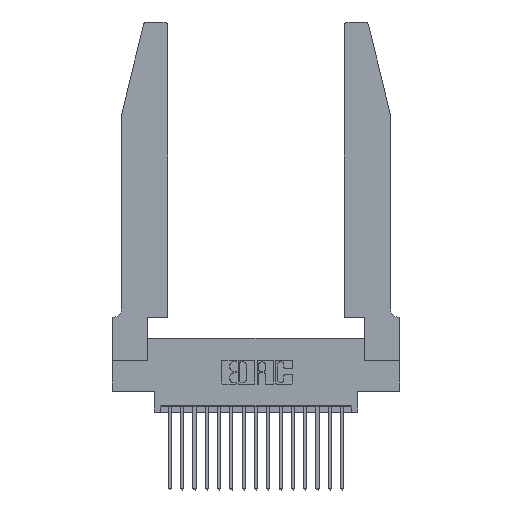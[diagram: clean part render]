
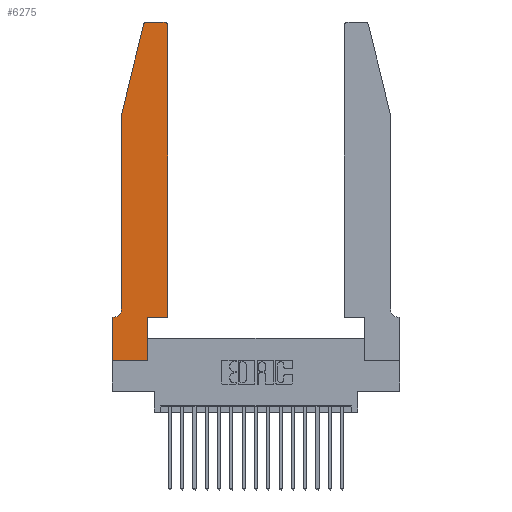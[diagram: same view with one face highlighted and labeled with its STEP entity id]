
A CAD part, top view. The second image highlights one B-rep face of the part: STEP entity #6275.
In plain terms, the highlighted planar face has unit normal (0, 0, 1).
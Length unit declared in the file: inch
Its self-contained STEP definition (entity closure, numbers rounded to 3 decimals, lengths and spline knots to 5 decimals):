
#132 = LINE ( 'NONE', #19241, #16407 ) ;
#251 = DIRECTION ( 'NONE',  ( -0.239, -0.971, 0. ) ) ;
#421 = ORIENTED_EDGE ( 'NONE', *, *, #3381, .T. ) ;
#512 = VECTOR ( 'NONE', #2416, 39.37008 ) ;
#868 = EDGE_CURVE ( 'NONE', #13616, #20068, #10272, .T. ) ;
#911 = ORIENTED_EDGE ( 'NONE', *, *, #13147, .T. ) ;
#1141 = EDGE_CURVE ( 'NONE', #5732, #8431, #18266, .T. ) ;
#1251 = CARTESIAN_POINT ( 'NONE',  ( 0.4205, 2.75, 0.37 ) ) ;
#1367 = VERTEX_POINT ( 'NONE', #13797 ) ;
#1369 = CARTESIAN_POINT ( 'NONE',  ( 0.4505, 0.35, 0.37 ) ) ;
#1503 = EDGE_CURVE ( 'NONE', #18216, #5732, #12931, .T. ) ;
#2416 = DIRECTION ( 'NONE',  ( 0., 1., 0. ) ) ;
#2422 = ORIENTED_EDGE ( 'NONE', *, *, #7272, .T. ) ;
#2637 = VERTEX_POINT ( 'NONE', #19944 ) ;
#2815 = CARTESIAN_POINT ( 'NONE',  ( 0.284, 2.75, 0.37 ) ) ;
#2861 = CARTESIAN_POINT ( 'NONE',  ( 0., 0.35, 0.37 ) ) ;
#2980 = VERTEX_POINT ( 'NONE', #4996 ) ;
#3059 = CARTESIAN_POINT ( 'NONE',  ( 0.0055, 0.42, 0.37 ) ) ;
#3167 = CARTESIAN_POINT ( 'NONE',  ( 0., 0.35, 0.37 ) ) ;
#3179 = ORIENTED_EDGE ( 'NONE', *, *, #16880, .T. ) ;
#3381 = EDGE_CURVE ( 'NONE', #19368, #2980, #3508, .T. ) ;
#3508 = LINE ( 'NONE', #18440, #19646 ) ;
#3659 = DIRECTION ( 'NONE',  ( 0., -1., 0. ) ) ;
#4074 = EDGE_CURVE ( 'NONE', #2980, #18216, #18404, .T. ) ;
#4141 = CARTESIAN_POINT ( 'NONE',  ( 0., 0., 0.37 ) ) ;
#4421 = ORIENTED_EDGE ( 'NONE', *, *, #868, .T. ) ;
#4464 = EDGE_CURVE ( 'NONE', #18987, #2637, #7931, .T. ) ;
#4649 = DIRECTION ( 'NONE',  ( -1., 0., 0. ) ) ;
#4820 = DIRECTION ( 'NONE',  ( 1., 0., 0. ) ) ;
#4996 = CARTESIAN_POINT ( 'NONE',  ( 0.4505, 2.72, 0.37 ) ) ;
#5023 = DIRECTION ( 'NONE',  ( 0., 0., 1. ) ) ;
#5327 = AXIS2_PLACEMENT_3D ( 'NONE', #14456, #5023, #15990 ) ;
#5559 = CARTESIAN_POINT ( 'NONE',  ( 0.0755, 0.35, 0.37 ) ) ;
#5666 = CARTESIAN_POINT ( 'NONE',  ( 0.2865, 0.35, 0.37 ) ) ;
#5732 = VERTEX_POINT ( 'NONE', #2815 ) ;
#6086 = PLANE ( 'NONE',  #13521 ) ;
#6092 = VECTOR ( 'NONE', #13229, 39.37008 ) ;
#6275 = ADVANCED_FACE ( 'NONE', ( #7425 ), #6086, .T. ) ;
#6898 = VECTOR ( 'NONE', #17969, 39.37008 ) ;
#7006 = EDGE_CURVE ( 'NONE', #8628, #19368, #7628, .T. ) ;
#7205 = CARTESIAN_POINT ( 'NONE',  ( 0.0755, 2., 0.37 ) ) ;
#7272 = EDGE_CURVE ( 'NONE', #2637, #13616, #19769, .T. ) ;
#7425 = FACE_OUTER_BOUND ( 'NONE', #13802, .T. ) ;
#7575 = DIRECTION ( 'NONE',  ( 0., 1., 0. ) ) ;
#7628 = LINE ( 'NONE', #1369, #20007 ) ;
#7666 = DIRECTION ( 'NONE',  ( 0., 0., 1. ) ) ;
#7931 = CIRCLE ( 'NONE', #10238, 0.07 ) ;
#8431 = VERTEX_POINT ( 'NONE', #14666 ) ;
#8628 = VERTEX_POINT ( 'NONE', #5666 ) ;
#8636 = CARTESIAN_POINT ( 'NONE',  ( 0.284, 2.72, 0.37 ) ) ;
#8788 = VECTOR ( 'NONE', #18674, 39.37008 ) ;
#8901 = ORIENTED_EDGE ( 'NONE', *, *, #4074, .T. ) ;
#9200 = DIRECTION ( 'NONE',  ( 0., 0., 1. ) ) ;
#10238 = AXIS2_PLACEMENT_3D ( 'NONE', #3059, #14094, #4649 ) ;
#10272 = LINE ( 'NONE', #15895, #6092 ) ;
#10351 = ORIENTED_EDGE ( 'NONE', *, *, #4464, .T. ) ;
#10864 = VECTOR ( 'NONE', #11062, 39.37008 ) ;
#10868 = DIRECTION ( 'NONE',  ( 1., 0., 0. ) ) ;
#11062 = DIRECTION ( 'NONE',  ( 1., 0., 0. ) ) ;
#11335 = LINE ( 'NONE', #12915, #19082 ) ;
#11890 = CARTESIAN_POINT ( 'NONE',  ( 0.2865, 0.35, 0.37 ) ) ;
#12915 = CARTESIAN_POINT ( 'NONE',  ( 0.0755, 2., 0.37 ) ) ;
#12931 = LINE ( 'NONE', #13414, #8788 ) ;
#13147 = EDGE_CURVE ( 'NONE', #8431, #14885, #11335, .T. ) ;
#13229 = DIRECTION ( 'NONE',  ( 0., -1., 0. ) ) ;
#13414 = CARTESIAN_POINT ( 'NONE',  ( 0.2605, 2.75, 0.37 ) ) ;
#13521 = AXIS2_PLACEMENT_3D ( 'NONE', #2861, #7666, #18542 ) ;
#13616 = VERTEX_POINT ( 'NONE', #3167 ) ;
#13797 = CARTESIAN_POINT ( 'NONE',  ( 0.2865, 0., 0.37 ) ) ;
#13802 = EDGE_LOOP ( 'NONE', ( #14254, #19310, #911, #14015, #10351, #2422, #4421, #17393, #3179, #16211, #421, #8901 ) ) ;
#13988 = EDGE_CURVE ( 'NONE', #14885, #18987, #132, .T. ) ;
#14015 = ORIENTED_EDGE ( 'NONE', *, *, #13988, .T. ) ;
#14094 = DIRECTION ( 'NONE',  ( 0., 0., -1. ) ) ;
#14254 = ORIENTED_EDGE ( 'NONE', *, *, #1503, .T. ) ;
#14456 = CARTESIAN_POINT ( 'NONE',  ( 0.4205, 2.72, 0.37 ) ) ;
#14666 = CARTESIAN_POINT ( 'NONE',  ( 0.25487, 2.72718, 0.37 ) ) ;
#14885 = VERTEX_POINT ( 'NONE', #7205 ) ;
#15014 = LINE ( 'NONE', #17228, #10864 ) ;
#15167 = AXIS2_PLACEMENT_3D ( 'NONE', #8636, #9200, #4820 ) ;
#15895 = CARTESIAN_POINT ( 'NONE',  ( 0., 0., 0.37 ) ) ;
#15990 = DIRECTION ( 'NONE',  ( 1., 0., 0. ) ) ;
#16211 = ORIENTED_EDGE ( 'NONE', *, *, #7006, .T. ) ;
#16299 = LINE ( 'NONE', #11890, #512 ) ;
#16407 = VECTOR ( 'NONE', #3659, 39.37008 ) ;
#16478 = CARTESIAN_POINT ( 'NONE',  ( 0.4505, 0.35, 0.37 ) ) ;
#16880 = EDGE_CURVE ( 'NONE', #1367, #8628, #16299, .T. ) ;
#17165 = CARTESIAN_POINT ( 'NONE',  ( 0.0755, 0.42, 0.37 ) ) ;
#17228 = CARTESIAN_POINT ( 'NONE',  ( 0., 0., 0.37 ) ) ;
#17393 = ORIENTED_EDGE ( 'NONE', *, *, #19805, .T. ) ;
#17969 = DIRECTION ( 'NONE',  ( -1., 0., 0. ) ) ;
#18216 = VERTEX_POINT ( 'NONE', #1251 ) ;
#18266 = CIRCLE ( 'NONE', #15167, 0.03 ) ;
#18404 = CIRCLE ( 'NONE', #5327, 0.03 ) ;
#18440 = CARTESIAN_POINT ( 'NONE',  ( 0.4505, 0.35, 0.37 ) ) ;
#18542 = DIRECTION ( 'NONE',  ( 1., 0., 0. ) ) ;
#18674 = DIRECTION ( 'NONE',  ( -1., 0., 0. ) ) ;
#18987 = VERTEX_POINT ( 'NONE', #17165 ) ;
#19082 = VECTOR ( 'NONE', #251, 39.37008 ) ;
#19241 = CARTESIAN_POINT ( 'NONE',  ( 0.0755, 2., 0.37 ) ) ;
#19310 = ORIENTED_EDGE ( 'NONE', *, *, #1141, .T. ) ;
#19368 = VERTEX_POINT ( 'NONE', #16478 ) ;
#19646 = VECTOR ( 'NONE', #7575, 39.37008 ) ;
#19769 = LINE ( 'NONE', #5559, #6898 ) ;
#19805 = EDGE_CURVE ( 'NONE', #20068, #1367, #15014, .T. ) ;
#19944 = CARTESIAN_POINT ( 'NONE',  ( 0.0055, 0.35, 0.37 ) ) ;
#20007 = VECTOR ( 'NONE', #10868, 39.37008 ) ;
#20068 = VERTEX_POINT ( 'NONE', #4141 ) ;
